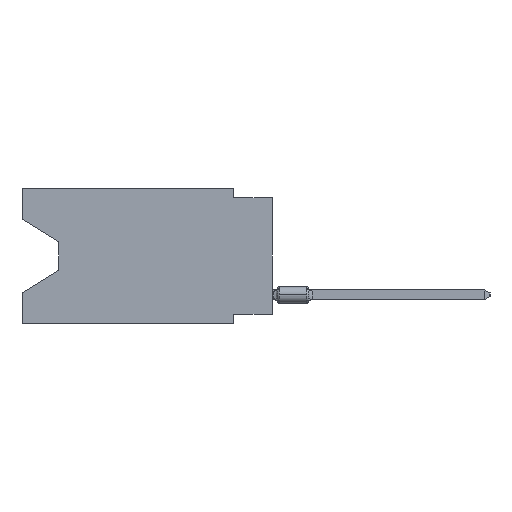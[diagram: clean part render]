
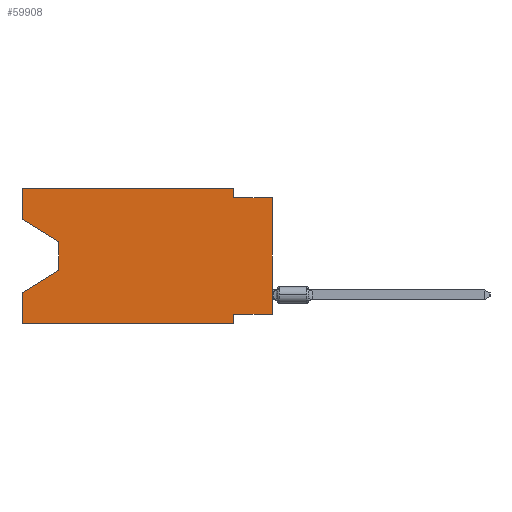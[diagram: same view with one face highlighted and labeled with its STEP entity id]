
A CAD part, left-side view. The second image highlights one B-rep face of the part: STEP entity #59908.
In plain terms, the highlighted planar face has unit normal (-1, 0, 0).
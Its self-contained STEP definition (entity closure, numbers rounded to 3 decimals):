
#4 = EDGE_CURVE ( 'NONE', #62556, #40658, #6433, .T. ) ;
#1444 = DIRECTION ( 'NONE',  ( 0., 0., 1. ) ) ;
#1646 = EDGE_CURVE ( 'NONE', #58090, #62556, #7653, .T. ) ;
#3916 = LINE ( 'NONE', #64762, #14472 ) ;
#4071 = CARTESIAN_POINT ( 'NONE',  ( 0., 0., -0.635 ) ) ;
#4813 = CARTESIAN_POINT ( 'NONE',  ( 0., 16.383, -2.038 ) ) ;
#5807 = DIRECTION ( 'NONE',  ( 0., 0., 1. ) ) ;
#6417 = VECTOR ( 'NONE', #19879, 1000. ) ;
#6433 = LINE ( 'NONE', #43867, #60595 ) ;
#6558 = DIRECTION ( 'NONE',  ( 0., 0., -1. ) ) ;
#6680 = VERTEX_POINT ( 'NONE', #13215 ) ;
#7215 = CARTESIAN_POINT ( 'NONE',  ( 0., 16.383, 0. ) ) ;
#7653 = LINE ( 'NONE', #59416, #68435 ) ;
#9484 = VECTOR ( 'NONE', #66849, 1000. ) ;
#9625 = VERTEX_POINT ( 'NONE', #37146 ) ;
#10150 = VECTOR ( 'NONE', #6558, 1000. ) ;
#10871 = EDGE_CURVE ( 'NONE', #40658, #44889, #51996, .T. ) ;
#10902 = VECTOR ( 'NONE', #21849, 1000. ) ;
#11070 = VERTEX_POINT ( 'NONE', #42908 ) ;
#13215 = CARTESIAN_POINT ( 'NONE',  ( 0., 2.54, -8.255 ) ) ;
#14472 = VECTOR ( 'NONE', #1444, 1000. ) ;
#14867 = LINE ( 'NONE', #57521, #10902 ) ;
#14921 = CARTESIAN_POINT ( 'NONE',  ( 0., 16.383, -8.89 ) ) ;
#16675 = PLANE ( 'NONE',  #50814 ) ;
#16922 = CARTESIAN_POINT ( 'NONE',  ( 0., 16.383, -6.852 ) ) ;
#17298 = DIRECTION ( 'NONE',  ( 0., 0., -1. ) ) ;
#17356 = LINE ( 'NONE', #61016, #46090 ) ;
#19339 = ORIENTED_EDGE ( 'NONE', *, *, #37793, .T. ) ;
#19879 = DIRECTION ( 'NONE',  ( 0., 1., 0. ) ) ;
#20110 = ORIENTED_EDGE ( 'NONE', *, *, #65369, .F. ) ;
#20524 = DIRECTION ( 'NONE',  ( 0., -1., 0. ) ) ;
#20875 = LINE ( 'NONE', #14921, #28272 ) ;
#21491 = CARTESIAN_POINT ( 'NONE',  ( 0., 2.54, 0. ) ) ;
#21849 = DIRECTION ( 'NONE',  ( 0., 0.855, -0.519 ) ) ;
#23940 = LINE ( 'NONE', #49230, #10150 ) ;
#23959 = VECTOR ( 'NONE', #5807, 1000. ) ;
#25137 = ORIENTED_EDGE ( 'NONE', *, *, #54399, .F. ) ;
#25469 = LINE ( 'NONE', #29340, #6417 ) ;
#27751 = VECTOR ( 'NONE', #62526, 1000. ) ;
#28272 = VECTOR ( 'NONE', #20524, 1000. ) ;
#29314 = DIRECTION ( 'NONE',  ( 0., -1., 0. ) ) ;
#29340 = CARTESIAN_POINT ( 'NONE',  ( 0., 0., -8.255 ) ) ;
#29729 = EDGE_CURVE ( 'NONE', #6680, #9625, #30031, .T. ) ;
#30031 = LINE ( 'NONE', #68480, #27751 ) ;
#30056 = ORIENTED_EDGE ( 'NONE', *, *, #29729, .F. ) ;
#31381 = VECTOR ( 'NONE', #29314, 1000. ) ;
#32108 = VERTEX_POINT ( 'NONE', #4813 ) ;
#32428 = DIRECTION ( 'NONE',  ( 0., 0., -1. ) ) ;
#33460 = FACE_OUTER_BOUND ( 'NONE', #37671, .T. ) ;
#35010 = CARTESIAN_POINT ( 'NONE',  ( 0., 13.97, -3.505 ) ) ;
#36835 = CARTESIAN_POINT ( 'NONE',  ( 0., 13.97, -5.385 ) ) ;
#37146 = CARTESIAN_POINT ( 'NONE',  ( 0., 2.54, -8.89 ) ) ;
#37658 = CARTESIAN_POINT ( 'NONE',  ( 0., 16.383, 0. ) ) ;
#37671 = EDGE_LOOP ( 'NONE', ( #64651, #57088, #67337, #66312, #47690, #30056, #20110, #19339, #40982, #54279, #42163, #25137 ) ) ;
#37793 = EDGE_CURVE ( 'NONE', #68940, #44889, #17356, .T. ) ;
#39538 = EDGE_CURVE ( 'NONE', #11070, #9625, #20875, .T. ) ;
#40658 = VERTEX_POINT ( 'NONE', #40821 ) ;
#40821 = CARTESIAN_POINT ( 'NONE',  ( 0., 2.54, -0.635 ) ) ;
#40982 = ORIENTED_EDGE ( 'NONE', *, *, #10871, .F. ) ;
#40987 = EDGE_CURVE ( 'NONE', #11070, #62587, #44268, .T. ) ;
#41748 = EDGE_CURVE ( 'NONE', #32108, #65046, #50427, .T. ) ;
#42163 = ORIENTED_EDGE ( 'NONE', *, *, #1646, .F. ) ;
#42908 = CARTESIAN_POINT ( 'NONE',  ( 0., 16.383, -8.89 ) ) ;
#43247 = DIRECTION ( 'NONE',  ( 1., 0., 0. ) ) ;
#43581 = CARTESIAN_POINT ( 'NONE',  ( 0., 16.383, 0. ) ) ;
#43867 = CARTESIAN_POINT ( 'NONE',  ( 0., 2.54, 0. ) ) ;
#44268 = LINE ( 'NONE', #37658, #23959 ) ;
#44889 = VERTEX_POINT ( 'NONE', #48857 ) ;
#45878 = EDGE_CURVE ( 'NONE', #54348, #62587, #14867, .T. ) ;
#46090 = VECTOR ( 'NONE', #49161, 1000. ) ;
#47056 = CARTESIAN_POINT ( 'NONE',  ( 0., 0., -8.255 ) ) ;
#47690 = ORIENTED_EDGE ( 'NONE', *, *, #39538, .T. ) ;
#48734 = EDGE_CURVE ( 'NONE', #65046, #54348, #23940, .T. ) ;
#48857 = CARTESIAN_POINT ( 'NONE',  ( 0., 0., -0.635 ) ) ;
#49161 = DIRECTION ( 'NONE',  ( 0., 0., 1. ) ) ;
#49230 = CARTESIAN_POINT ( 'NONE',  ( 0., 13.97, -3.505 ) ) ;
#50427 = LINE ( 'NONE', #65474, #9484 ) ;
#50814 = AXIS2_PLACEMENT_3D ( 'NONE', #43581, #43247, #32428 ) ;
#51996 = LINE ( 'NONE', #4071, #31381 ) ;
#54279 = ORIENTED_EDGE ( 'NONE', *, *, #4, .F. ) ;
#54348 = VERTEX_POINT ( 'NONE', #36835 ) ;
#54399 = EDGE_CURVE ( 'NONE', #32108, #58090, #3916, .T. ) ;
#55555 = DIRECTION ( 'NONE',  ( 0., -1., 0. ) ) ;
#57088 = ORIENTED_EDGE ( 'NONE', *, *, #48734, .T. ) ;
#57521 = CARTESIAN_POINT ( 'NONE',  ( 0., 13.97, -5.385 ) ) ;
#58090 = VERTEX_POINT ( 'NONE', #7215 ) ;
#59416 = CARTESIAN_POINT ( 'NONE',  ( 0., 16.383, 0. ) ) ;
#59908 = ADVANCED_FACE ( 'NONE', ( #33460 ), #16675, .F. ) ;
#60595 = VECTOR ( 'NONE', #17298, 1000. ) ;
#61016 = CARTESIAN_POINT ( 'NONE',  ( 0., 0., 0. ) ) ;
#62526 = DIRECTION ( 'NONE',  ( 0., 0., -1. ) ) ;
#62556 = VERTEX_POINT ( 'NONE', #21491 ) ;
#62587 = VERTEX_POINT ( 'NONE', #16922 ) ;
#64651 = ORIENTED_EDGE ( 'NONE', *, *, #41748, .T. ) ;
#64762 = CARTESIAN_POINT ( 'NONE',  ( 0., 16.383, 0. ) ) ;
#65046 = VERTEX_POINT ( 'NONE', #35010 ) ;
#65369 = EDGE_CURVE ( 'NONE', #68940, #6680, #25469, .T. ) ;
#65474 = CARTESIAN_POINT ( 'NONE',  ( 0., 16.383, -2.038 ) ) ;
#66312 = ORIENTED_EDGE ( 'NONE', *, *, #40987, .F. ) ;
#66849 = DIRECTION ( 'NONE',  ( 0., -0.855, -0.519 ) ) ;
#67337 = ORIENTED_EDGE ( 'NONE', *, *, #45878, .T. ) ;
#68435 = VECTOR ( 'NONE', #55555, 1000. ) ;
#68480 = CARTESIAN_POINT ( 'NONE',  ( 0., 2.54, -8.89 ) ) ;
#68940 = VERTEX_POINT ( 'NONE', #47056 ) ;
